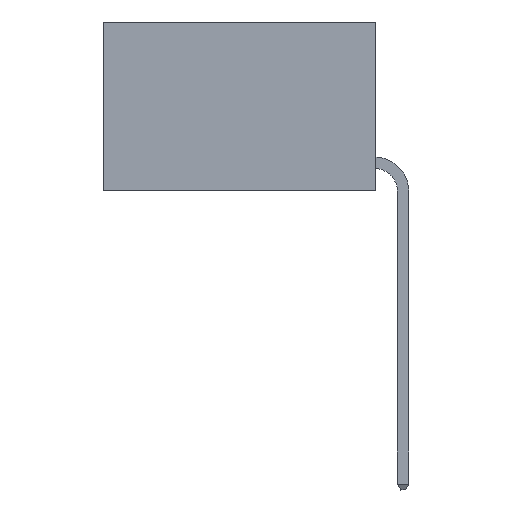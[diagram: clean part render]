
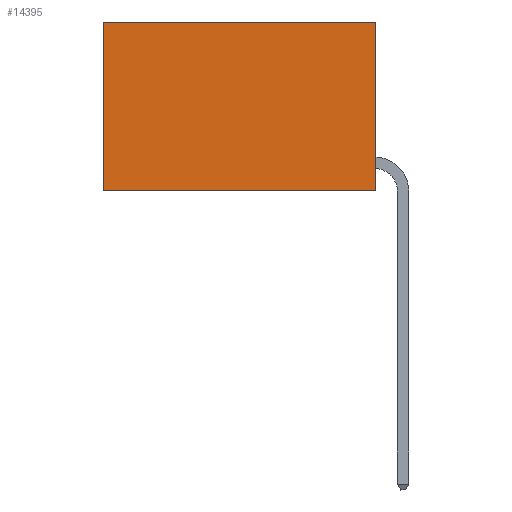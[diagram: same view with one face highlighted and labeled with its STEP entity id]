
A CAD part, left-side view. The second image highlights one B-rep face of the part: STEP entity #14395.
In plain terms, the highlighted planar face has unit normal (-1, 0, 0).
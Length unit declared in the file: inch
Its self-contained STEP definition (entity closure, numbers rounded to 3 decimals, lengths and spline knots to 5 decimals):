
#1006 = VERTEX_POINT ( 'NONE', #13761 ) ;
#1602 = VECTOR ( 'NONE', #5835, 39.37008 ) ;
#1615 = VERTEX_POINT ( 'NONE', #5001 ) ;
#2347 = LINE ( 'NONE', #10479, #10507 ) ;
#3106 = VERTEX_POINT ( 'NONE', #7044 ) ;
#3685 = DIRECTION ( 'NONE',  ( 0., 0., -1. ) ) ;
#4323 = EDGE_CURVE ( 'NONE', #3106, #1006, #11099, .T. ) ;
#5001 = CARTESIAN_POINT ( 'NONE',  ( 0.2625, 0., 0. ) ) ;
#5644 = CARTESIAN_POINT ( 'NONE',  ( 0.2625, 0.6, 0. ) ) ;
#5835 = DIRECTION ( 'NONE',  ( 0., 0., -1. ) ) ;
#7044 = CARTESIAN_POINT ( 'NONE',  ( 0.2625, 0., -0.37 ) ) ;
#7394 = LINE ( 'NONE', #5644, #1602 ) ;
#7483 = DIRECTION ( 'NONE',  ( 0., 1., 0. ) ) ;
#8517 = FACE_OUTER_BOUND ( 'NONE', #12438, .T. ) ;
#9257 = CARTESIAN_POINT ( 'NONE',  ( 0.2625, 0., 0. ) ) ;
#10479 = CARTESIAN_POINT ( 'NONE',  ( 0.2625, 0., 0. ) ) ;
#10507 = VECTOR ( 'NONE', #7483, 39.37008 ) ;
#11057 = ORIENTED_EDGE ( 'NONE', *, *, #18715, .F. ) ;
#11099 = LINE ( 'NONE', #15815, #14937 ) ;
#11360 = EDGE_CURVE ( 'NONE', #1615, #13149, #2347, .T. ) ;
#11382 = EDGE_CURVE ( 'NONE', #13149, #1006, #7394, .T. ) ;
#11935 = CARTESIAN_POINT ( 'NONE',  ( 0.2625, 0., 0. ) ) ;
#11954 = LINE ( 'NONE', #9257, #19275 ) ;
#12125 = CARTESIAN_POINT ( 'NONE',  ( 0.2625, 0.6, 0. ) ) ;
#12438 = EDGE_LOOP ( 'NONE', ( #13147, #13331, #11057, #20388 ) ) ;
#13147 = ORIENTED_EDGE ( 'NONE', *, *, #11382, .T. ) ;
#13149 = VERTEX_POINT ( 'NONE', #12125 ) ;
#13331 = ORIENTED_EDGE ( 'NONE', *, *, #4323, .F. ) ;
#13761 = CARTESIAN_POINT ( 'NONE',  ( 0.2625, 0.6, -0.37 ) ) ;
#14139 = DIRECTION ( 'NONE',  ( 0., 1., 0. ) ) ;
#14395 = ADVANCED_FACE ( 'NONE', ( #8517 ), #17914, .F. ) ;
#14507 = AXIS2_PLACEMENT_3D ( 'NONE', #11935, #18323, #3685 ) ;
#14937 = VECTOR ( 'NONE', #14139, 39.37008 ) ;
#15815 = CARTESIAN_POINT ( 'NONE',  ( 0.2625, 0., -0.37 ) ) ;
#16777 = DIRECTION ( 'NONE',  ( 0., 0., -1. ) ) ;
#17914 = PLANE ( 'NONE',  #14507 ) ;
#18323 = DIRECTION ( 'NONE',  ( 1., 0., 0. ) ) ;
#18715 = EDGE_CURVE ( 'NONE', #1615, #3106, #11954, .T. ) ;
#19275 = VECTOR ( 'NONE', #16777, 39.37008 ) ;
#20388 = ORIENTED_EDGE ( 'NONE', *, *, #11360, .T. ) ;
